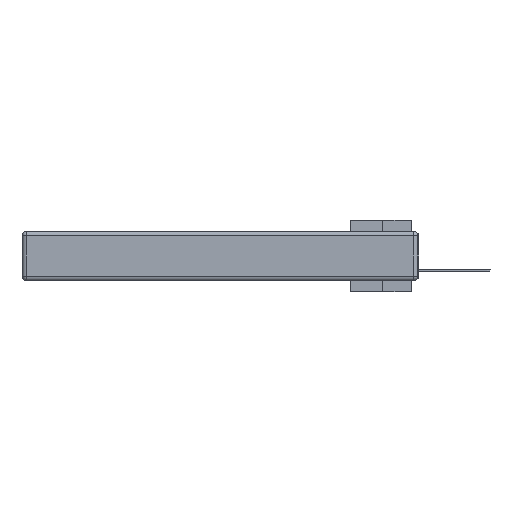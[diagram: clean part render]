
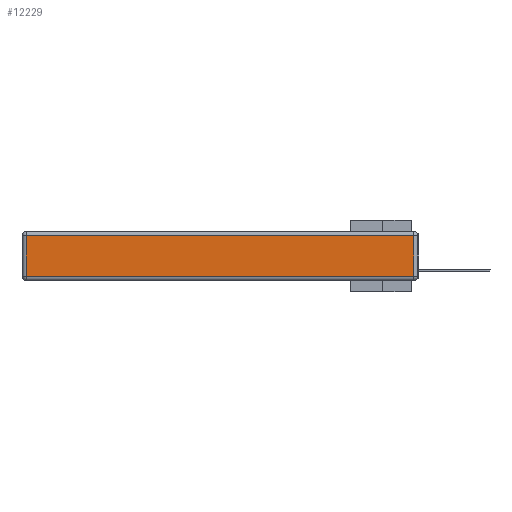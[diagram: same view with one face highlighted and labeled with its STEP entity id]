
A CAD part, left-side view. The second image highlights one B-rep face of the part: STEP entity #12229.
In plain terms, the highlighted planar face has unit normal (-1, 0, 0).
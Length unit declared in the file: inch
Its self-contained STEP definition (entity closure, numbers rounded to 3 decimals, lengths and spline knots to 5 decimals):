
#500 = EDGE_CURVE ( 'NONE', #7433, #8790, #30576, .T. ) ;
#1073 = ORIENTED_EDGE ( 'NONE', *, *, #500, .T. ) ;
#1239 = DIRECTION ( 'NONE',  ( 0., 0., 1. ) ) ;
#1445 = CARTESIAN_POINT ( 'NONE',  ( 0., 0.03, -0.313 ) ) ;
#1473 = EDGE_CURVE ( 'NONE', #8790, #2629, #19490, .T. ) ;
#2052 = LINE ( 'NONE', #8907, #10449 ) ;
#2629 = VERTEX_POINT ( 'NONE', #1445 ) ;
#3011 = DIRECTION ( 'NONE',  ( 0., 0., 1. ) ) ;
#7325 = DIRECTION ( 'NONE',  ( 0., -1., 0. ) ) ;
#7433 = VERTEX_POINT ( 'NONE', #10214 ) ;
#8138 = DIRECTION ( 'NONE',  ( 0., 0., -1. ) ) ;
#8331 = EDGE_CURVE ( 'NONE', #11786, #7433, #2052, .T. ) ;
#8790 = VERTEX_POINT ( 'NONE', #18208 ) ;
#8907 = CARTESIAN_POINT ( 'NONE',  ( 0., 2.75, -0.03 ) ) ;
#10214 = CARTESIAN_POINT ( 'NONE',  ( 0., 2.72, -0.03 ) ) ;
#10302 = CARTESIAN_POINT ( 'NONE',  ( 0., 0.03, -0.03 ) ) ;
#10449 = VECTOR ( 'NONE', #19968, 39.37008 ) ;
#11667 = ORIENTED_EDGE ( 'NONE', *, *, #18755, .T. ) ;
#11786 = VERTEX_POINT ( 'NONE', #10302 ) ;
#11970 = VECTOR ( 'NONE', #7325, 39.37008 ) ;
#12229 = ADVANCED_FACE ( 'NONE', ( #20341 ), #29205, .T. ) ;
#12850 = ORIENTED_EDGE ( 'NONE', *, *, #8331, .T. ) ;
#17083 = CARTESIAN_POINT ( 'NONE',  ( 0., 0.03, -0.343 ) ) ;
#18208 = CARTESIAN_POINT ( 'NONE',  ( 0., 2.72, -0.313 ) ) ;
#18332 = VECTOR ( 'NONE', #3011, 39.37008 ) ;
#18552 = CARTESIAN_POINT ( 'NONE',  ( 0., 0., -0.313 ) ) ;
#18755 = EDGE_CURVE ( 'NONE', #2629, #11786, #23152, .T. ) ;
#19490 = LINE ( 'NONE', #18552, #11970 ) ;
#19968 = DIRECTION ( 'NONE',  ( 0., 1., 0. ) ) ;
#20341 = FACE_OUTER_BOUND ( 'NONE', #25215, .T. ) ;
#22176 = CARTESIAN_POINT ( 'NONE',  ( 0., 2.72, -0.343 ) ) ;
#23085 = VECTOR ( 'NONE', #8138, 39.37008 ) ;
#23152 = LINE ( 'NONE', #17083, #18332 ) ;
#25215 = EDGE_LOOP ( 'NONE', ( #35973, #11667, #12850, #1073 ) ) ;
#29205 = PLANE ( 'NONE',  #35936 ) ;
#30576 = LINE ( 'NONE', #22176, #23085 ) ;
#32586 = DIRECTION ( 'NONE',  ( -1., 0., 0. ) ) ;
#35149 = CARTESIAN_POINT ( 'NONE',  ( 0., 0., -0.343 ) ) ;
#35936 = AXIS2_PLACEMENT_3D ( 'NONE', #35149, #32586, #1239 ) ;
#35973 = ORIENTED_EDGE ( 'NONE', *, *, #1473, .T. ) ;
